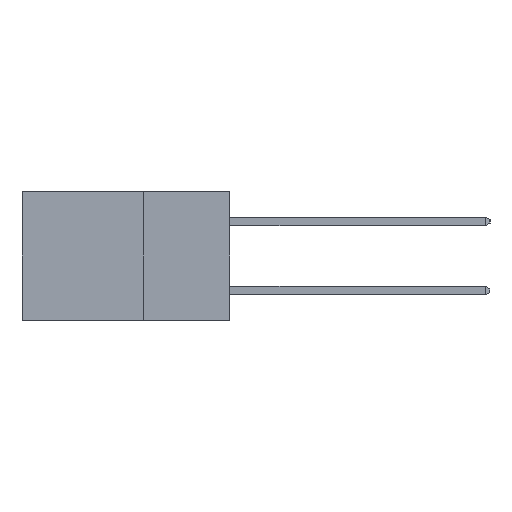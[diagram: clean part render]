
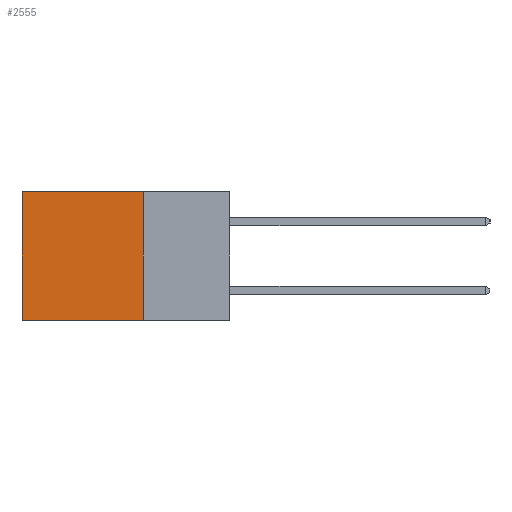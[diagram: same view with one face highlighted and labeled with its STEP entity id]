
A CAD part, left-side view. The second image highlights one B-rep face of the part: STEP entity #2555.
In plain terms, the highlighted planar face has unit normal (-1, 0, 0).
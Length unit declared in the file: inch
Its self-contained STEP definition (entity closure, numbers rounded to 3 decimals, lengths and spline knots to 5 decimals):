
#219 = EDGE_CURVE ( 'NONE', #5254, #5692, #7123, .T. ) ;
#513 = LINE ( 'NONE', #9646, #10122 ) ;
#617 = FACE_OUTER_BOUND ( 'NONE', #2049, .T. ) ;
#686 = EDGE_CURVE ( 'NONE', #5254, #10576, #6185, .T. ) ;
#1083 = EDGE_CURVE ( 'NONE', #5692, #11667, #513, .T. ) ;
#1149 = CARTESIAN_POINT ( 'NONE',  ( 0.298, 0.25, 0. ) ) ;
#1372 = LINE ( 'NONE', #7975, #3550 ) ;
#1493 = DIRECTION ( 'NONE',  ( 0., 1., 0. ) ) ;
#1783 = PLANE ( 'NONE',  #10214 ) ;
#2049 = EDGE_LOOP ( 'NONE', ( #3929, #3963, #3966, #4079 ) ) ;
#2118 = CARTESIAN_POINT ( 'NONE',  ( 0.298, 0.25, 0. ) ) ;
#2198 = DIRECTION ( 'NONE',  ( 0., 1., 0. ) ) ;
#2555 = ADVANCED_FACE ( 'NONE', ( #617 ), #1783, .F. ) ;
#2748 = CARTESIAN_POINT ( 'NONE',  ( 0.298, 0.25, 0. ) ) ;
#3550 = VECTOR ( 'NONE', #2198, 39.37008 ) ;
#3929 = ORIENTED_EDGE ( 'NONE', *, *, #1083, .T. ) ;
#3963 = ORIENTED_EDGE ( 'NONE', *, *, #11773, .F. ) ;
#3966 = ORIENTED_EDGE ( 'NONE', *, *, #686, .F. ) ;
#4069 = DIRECTION ( 'NONE',  ( 1., 0., 0. ) ) ;
#4079 = ORIENTED_EDGE ( 'NONE', *, *, #219, .T. ) ;
#4401 = DIRECTION ( 'NONE',  ( 0., 0., -1. ) ) ;
#4778 = CARTESIAN_POINT ( 'NONE',  ( 0.298, 0.25, 0. ) ) ;
#5254 = VERTEX_POINT ( 'NONE', #4778 ) ;
#5692 = VERTEX_POINT ( 'NONE', #11174 ) ;
#6185 = LINE ( 'NONE', #1149, #7433 ) ;
#7123 = LINE ( 'NONE', #2118, #11830 ) ;
#7433 = VECTOR ( 'NONE', #4401, 39.37008 ) ;
#7772 = CARTESIAN_POINT ( 'NONE',  ( 0.298, 0.6, -0.37 ) ) ;
#7975 = CARTESIAN_POINT ( 'NONE',  ( 0.298, 0.25, -0.37 ) ) ;
#7987 = DIRECTION ( 'NONE',  ( 0., 0., -1. ) ) ;
#8143 = DIRECTION ( 'NONE',  ( 0., 0., -1. ) ) ;
#9646 = CARTESIAN_POINT ( 'NONE',  ( 0.298, 0.6, 0. ) ) ;
#10013 = CARTESIAN_POINT ( 'NONE',  ( 0.298, 0.25, -0.37 ) ) ;
#10122 = VECTOR ( 'NONE', #7987, 39.37008 ) ;
#10214 = AXIS2_PLACEMENT_3D ( 'NONE', #2748, #4069, #8143 ) ;
#10576 = VERTEX_POINT ( 'NONE', #10013 ) ;
#11174 = CARTESIAN_POINT ( 'NONE',  ( 0.298, 0.6, 0. ) ) ;
#11667 = VERTEX_POINT ( 'NONE', #7772 ) ;
#11773 = EDGE_CURVE ( 'NONE', #10576, #11667, #1372, .T. ) ;
#11830 = VECTOR ( 'NONE', #1493, 39.37008 ) ;
